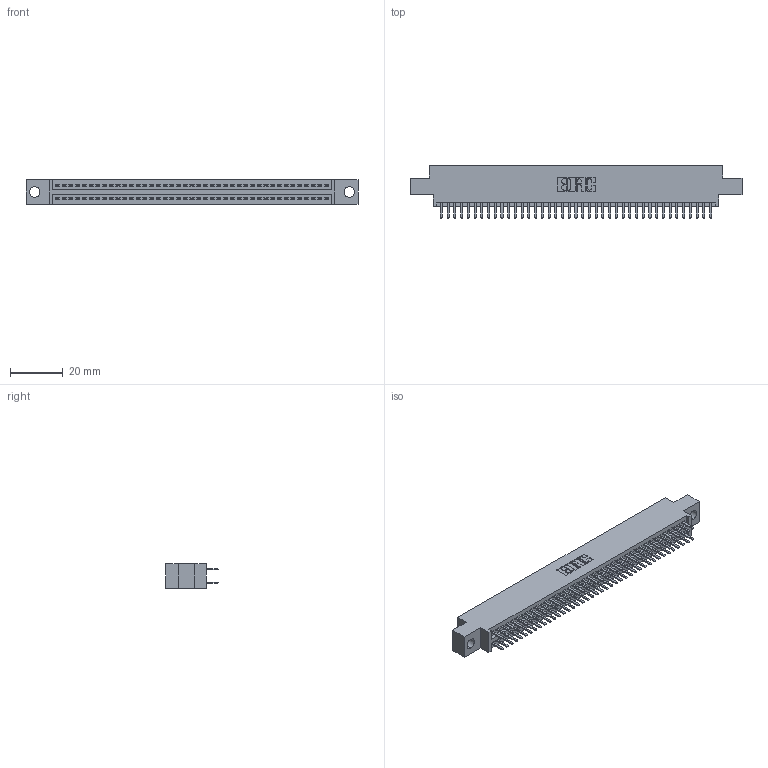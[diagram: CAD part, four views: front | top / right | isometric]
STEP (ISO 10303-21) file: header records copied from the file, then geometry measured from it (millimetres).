
FILE_DESCRIPTION (( 'STEP AP203' ), '1' );
FILE_NAME ('395-082-520-804.STEP', '2021-06-17T07:31:30', ( '' ), ( '' ), 'SwSTEP 2.0', 'SolidWorks 2020', '' );
FILE_SCHEMA (( 'CONFIG_CONTROL_DESIGN' ));
Length unit declared in the file: inch
Products named in the file (3): 345-292-001_345-293-120; 395-082-520-804; 345 Part_0.170 Offset - 0.156 Dia-TI
Assembly tree (83 placements, depth 2):
  395-082-520-804
    345 Part_0.170 Offset - 0.156 Dia-TI
    345-292-001_345-293-120  x82
Bounding box: 125.35 x 19.68 x 9.4 mm (x, y, z)
Volume: 11911.9 mm3; surface area: 17506.8 mm2
Topology: 83 solids, 83 shells, 4572 faces, 13263 edges, 8622 vertices
Faces by surface type: plane 2968, cylinder 1604
Entity records: 32969 total; most frequent: CARTESIAN_POINT 5546, ORIENTED_EDGE 5466, DIRECTION 4877, EDGE_CURVE 2733, LINE 2433, VECTOR 2433, VERTEX_POINT 1818, AXIS2_PLACEMENT_3D 1222
